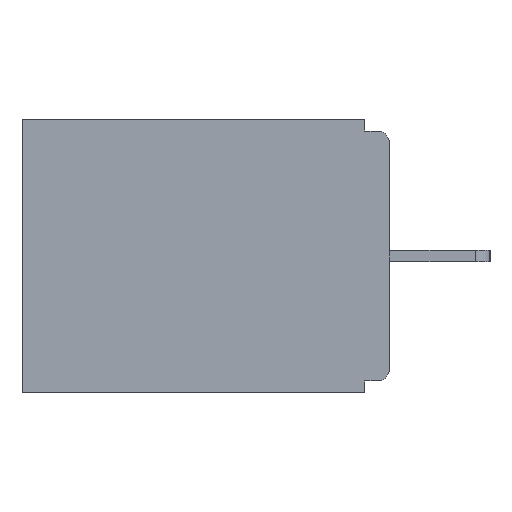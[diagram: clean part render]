
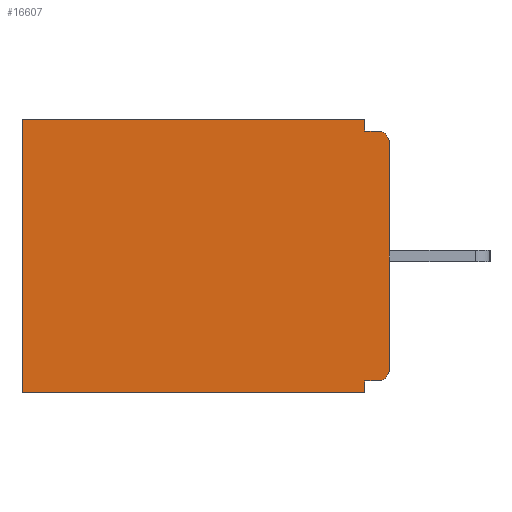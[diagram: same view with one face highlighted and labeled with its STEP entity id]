
A CAD part, left-side view. The second image highlights one B-rep face of the part: STEP entity #16607.
In plain terms, the highlighted planar face has unit normal (-1, 0, 0).
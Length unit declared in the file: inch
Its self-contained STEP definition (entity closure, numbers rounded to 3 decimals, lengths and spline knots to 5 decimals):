
#689 = ORIENTED_EDGE ( 'NONE', *, *, #4437, .T. ) ;
#712 = LINE ( 'NONE', #13733, #17833 ) ;
#882 = LINE ( 'NONE', #21662, #9604 ) ;
#992 = CARTESIAN_POINT ( 'NONE',  ( 0.298, 0.46, 0. ) ) ;
#1373 = CARTESIAN_POINT ( 'NONE',  ( 0.298, 0., 0. ) ) ;
#1487 = CARTESIAN_POINT ( 'NONE',  ( 0.298, 0., -0.313 ) ) ;
#1829 = VERTEX_POINT ( 'NONE', #18679 ) ;
#1845 = CARTESIAN_POINT ( 'NONE',  ( 0.298, 0.031, -0.328 ) ) ;
#1885 = CIRCLE ( 'NONE', #10045, 0.015 ) ;
#1948 = CARTESIAN_POINT ( 'NONE',  ( 0.298, 0.46, -0.343 ) ) ;
#1974 = VERTEX_POINT ( 'NONE', #4749 ) ;
#2002 = VECTOR ( 'NONE', #21263, 39.37008 ) ;
#2026 = VERTEX_POINT ( 'NONE', #6198 ) ;
#2097 = ORIENTED_EDGE ( 'NONE', *, *, #12133, .F. ) ;
#2099 = DIRECTION ( 'NONE',  ( -1., 0., 0. ) ) ;
#2957 = CARTESIAN_POINT ( 'NONE',  ( 0.298, 0., -0.03 ) ) ;
#3255 = CARTESIAN_POINT ( 'NONE',  ( 0.298, 0.46, 0. ) ) ;
#3335 = EDGE_CURVE ( 'NONE', #1829, #9383, #14949, .T. ) ;
#3389 = EDGE_CURVE ( 'NONE', #15924, #9383, #5331, .T. ) ;
#3558 = EDGE_CURVE ( 'NONE', #12029, #16041, #5583, .T. ) ;
#4236 = CARTESIAN_POINT ( 'NONE',  ( 0.298, 0., -0.328 ) ) ;
#4437 = EDGE_CURVE ( 'NONE', #16041, #13066, #6060, .T. ) ;
#4749 = CARTESIAN_POINT ( 'NONE',  ( 0.298, 0.015, -0.015 ) ) ;
#5146 = CARTESIAN_POINT ( 'NONE',  ( 0.298, 0., -0.015 ) ) ;
#5331 = LINE ( 'NONE', #19935, #17769 ) ;
#5425 = EDGE_CURVE ( 'NONE', #9164, #1974, #11966, .T. ) ;
#5583 = LINE ( 'NONE', #14834, #19032 ) ;
#5833 = VECTOR ( 'NONE', #5958, 39.37008 ) ;
#5958 = DIRECTION ( 'NONE',  ( 0., 1., 0. ) ) ;
#6060 = LINE ( 'NONE', #992, #2002 ) ;
#6198 = CARTESIAN_POINT ( 'NONE',  ( 0.298, 0.031, -0.343 ) ) ;
#6582 = VECTOR ( 'NONE', #7555, 39.37008 ) ;
#6615 = PLANE ( 'NONE',  #6783 ) ;
#6663 = DIRECTION ( 'NONE',  ( 0., 1., 0. ) ) ;
#6677 = ORIENTED_EDGE ( 'NONE', *, *, #3389, .F. ) ;
#6783 = AXIS2_PLACEMENT_3D ( 'NONE', #1373, #18407, #8370 ) ;
#7060 = EDGE_LOOP ( 'NONE', ( #15953, #20280, #2097, #21116, #689, #7741, #18688, #20670, #19653, #6677 ) ) ;
#7555 = DIRECTION ( 'NONE',  ( 0., 1., 0. ) ) ;
#7733 = CARTESIAN_POINT ( 'NONE',  ( 0.298, 0.015, -0.313 ) ) ;
#7741 = ORIENTED_EDGE ( 'NONE', *, *, #9569, .F. ) ;
#8370 = DIRECTION ( 'NONE',  ( 0., 0., -1. ) ) ;
#8442 = DIRECTION ( 'NONE',  ( 0., -1., 0. ) ) ;
#8587 = DIRECTION ( 'NONE',  ( 0., 0., -1. ) ) ;
#9164 = VERTEX_POINT ( 'NONE', #12047 ) ;
#9383 = VERTEX_POINT ( 'NONE', #1487 ) ;
#9548 = DIRECTION ( 'NONE',  ( -1., 0., 0. ) ) ;
#9569 = EDGE_CURVE ( 'NONE', #2026, #13066, #11197, .T. ) ;
#9604 = VECTOR ( 'NONE', #11750, 39.37008 ) ;
#10045 = AXIS2_PLACEMENT_3D ( 'NONE', #19527, #9548, #21152 ) ;
#11197 = LINE ( 'NONE', #20169, #6582 ) ;
#11497 = LINE ( 'NONE', #4236, #5833 ) ;
#11750 = DIRECTION ( 'NONE',  ( 0., 0., -1. ) ) ;
#11966 = LINE ( 'NONE', #5146, #15905 ) ;
#12029 = VERTEX_POINT ( 'NONE', #18337 ) ;
#12047 = CARTESIAN_POINT ( 'NONE',  ( 0.298, 0.031, -0.015 ) ) ;
#12133 = EDGE_CURVE ( 'NONE', #12029, #9164, #712, .T. ) ;
#13066 = VERTEX_POINT ( 'NONE', #1948 ) ;
#13733 = CARTESIAN_POINT ( 'NONE',  ( 0.298, 0.031, -0.343 ) ) ;
#14834 = CARTESIAN_POINT ( 'NONE',  ( 0.298, 0., 0. ) ) ;
#14949 = CIRCLE ( 'NONE', #16556, 0.015 ) ;
#15155 = FACE_OUTER_BOUND ( 'NONE', #7060, .T. ) ;
#15905 = VECTOR ( 'NONE', #8442, 39.37008 ) ;
#15924 = VERTEX_POINT ( 'NONE', #2957 ) ;
#15953 = ORIENTED_EDGE ( 'NONE', *, *, #20342, .T. ) ;
#16041 = VERTEX_POINT ( 'NONE', #3255 ) ;
#16384 = EDGE_CURVE ( 'NONE', #1829, #16745, #11497, .T. ) ;
#16556 = AXIS2_PLACEMENT_3D ( 'NONE', #7733, #2099, #19007 ) ;
#16607 = ADVANCED_FACE ( 'NONE', ( #15155 ), #6615, .F. ) ;
#16644 = EDGE_CURVE ( 'NONE', #16745, #2026, #882, .T. ) ;
#16745 = VERTEX_POINT ( 'NONE', #1845 ) ;
#17769 = VECTOR ( 'NONE', #18972, 39.37008 ) ;
#17833 = VECTOR ( 'NONE', #8587, 39.37008 ) ;
#18337 = CARTESIAN_POINT ( 'NONE',  ( 0.298, 0.031, 0. ) ) ;
#18407 = DIRECTION ( 'NONE',  ( 1., 0., 0. ) ) ;
#18679 = CARTESIAN_POINT ( 'NONE',  ( 0.298, 0.015, -0.328 ) ) ;
#18688 = ORIENTED_EDGE ( 'NONE', *, *, #16644, .F. ) ;
#18972 = DIRECTION ( 'NONE',  ( 0., 0., -1. ) ) ;
#19007 = DIRECTION ( 'NONE',  ( 0., 0., -1. ) ) ;
#19032 = VECTOR ( 'NONE', #6663, 39.37008 ) ;
#19527 = CARTESIAN_POINT ( 'NONE',  ( 0.298, 0.015, -0.03 ) ) ;
#19653 = ORIENTED_EDGE ( 'NONE', *, *, #3335, .T. ) ;
#19935 = CARTESIAN_POINT ( 'NONE',  ( 0.298, 0., 0. ) ) ;
#20169 = CARTESIAN_POINT ( 'NONE',  ( 0.298, 0., -0.343 ) ) ;
#20280 = ORIENTED_EDGE ( 'NONE', *, *, #5425, .F. ) ;
#20342 = EDGE_CURVE ( 'NONE', #15924, #1974, #1885, .T. ) ;
#20670 = ORIENTED_EDGE ( 'NONE', *, *, #16384, .F. ) ;
#21116 = ORIENTED_EDGE ( 'NONE', *, *, #3558, .T. ) ;
#21152 = DIRECTION ( 'NONE',  ( 0., 0., -1. ) ) ;
#21263 = DIRECTION ( 'NONE',  ( 0., 0., -1. ) ) ;
#21662 = CARTESIAN_POINT ( 'NONE',  ( 0.298, 0.031, -0.343 ) ) ;
